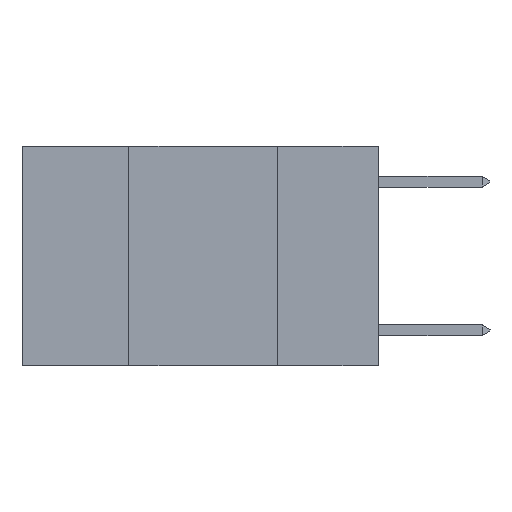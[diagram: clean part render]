
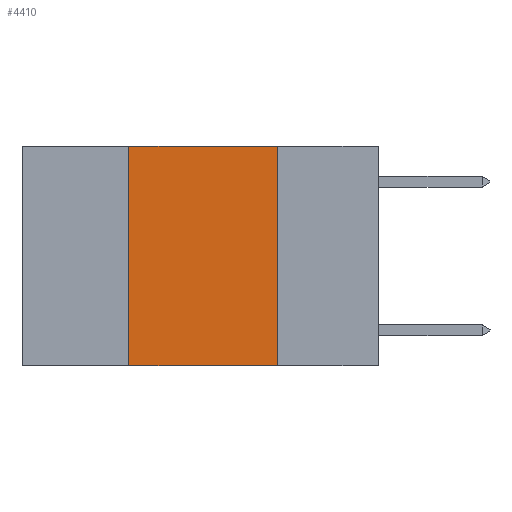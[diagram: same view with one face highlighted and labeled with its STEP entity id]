
A CAD part, left-side view. The second image highlights one B-rep face of the part: STEP entity #4410.
In plain terms, the highlighted planar face has unit normal (-1, 0, 0).
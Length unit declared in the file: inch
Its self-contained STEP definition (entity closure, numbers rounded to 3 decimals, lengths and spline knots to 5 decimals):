
#811 = VERTEX_POINT ( 'NONE', #2600 ) ;
#823 = DIRECTION ( 'NONE',  ( 0., 0., -1. ) ) ;
#842 = VECTOR ( 'NONE', #6022, 39.37008 ) ;
#880 = AXIS2_PLACEMENT_3D ( 'NONE', #5152, #6126, #823 ) ;
#996 = LINE ( 'NONE', #3697, #5371 ) ;
#1858 = VECTOR ( 'NONE', #10488, 39.37008 ) ;
#2410 = VECTOR ( 'NONE', #9389, 39.37008 ) ;
#2423 = VERTEX_POINT ( 'NONE', #10660 ) ;
#2434 = EDGE_CURVE ( 'NONE', #2423, #6472, #996, .T. ) ;
#2500 = EDGE_CURVE ( 'NONE', #811, #2423, #2654, .T. ) ;
#2600 = CARTESIAN_POINT ( 'NONE',  ( 0., 0.42, -0.37 ) ) ;
#2654 = LINE ( 'NONE', #4223, #2410 ) ;
#2968 = VERTEX_POINT ( 'NONE', #3787 ) ;
#3271 = EDGE_CURVE ( 'NONE', #811, #2968, #7727, .T. ) ;
#3697 = CARTESIAN_POINT ( 'NONE',  ( 0., 0.6, 0. ) ) ;
#3787 = CARTESIAN_POINT ( 'NONE',  ( 0., 0.17, -0.37 ) ) ;
#4223 = CARTESIAN_POINT ( 'NONE',  ( 0., 0.42, 0. ) ) ;
#4410 = ADVANCED_FACE ( 'NONE', ( #5024 ), #8493, .F. ) ;
#5024 = FACE_OUTER_BOUND ( 'NONE', #6814, .T. ) ;
#5152 = CARTESIAN_POINT ( 'NONE',  ( 0., 0.6, 0. ) ) ;
#5371 = VECTOR ( 'NONE', #9566, 39.37008 ) ;
#6022 = DIRECTION ( 'NONE',  ( 0., -1., 0. ) ) ;
#6126 = DIRECTION ( 'NONE',  ( 1., 0., 0. ) ) ;
#6472 = VERTEX_POINT ( 'NONE', #7845 ) ;
#6723 = EDGE_CURVE ( 'NONE', #6472, #2968, #10813, .T. ) ;
#6814 = EDGE_LOOP ( 'NONE', ( #9332, #8508, #8942, #9829 ) ) ;
#7570 = CARTESIAN_POINT ( 'NONE',  ( 0., 0.6, -0.37 ) ) ;
#7727 = LINE ( 'NONE', #7570, #842 ) ;
#7845 = CARTESIAN_POINT ( 'NONE',  ( 0., 0.17, 0. ) ) ;
#8493 = PLANE ( 'NONE',  #880 ) ;
#8508 = ORIENTED_EDGE ( 'NONE', *, *, #2434, .F. ) ;
#8942 = ORIENTED_EDGE ( 'NONE', *, *, #2500, .F. ) ;
#9332 = ORIENTED_EDGE ( 'NONE', *, *, #6723, .F. ) ;
#9389 = DIRECTION ( 'NONE',  ( 0., 0., 1. ) ) ;
#9566 = DIRECTION ( 'NONE',  ( 0., -1., 0. ) ) ;
#9713 = CARTESIAN_POINT ( 'NONE',  ( 0., 0.17, 0. ) ) ;
#9829 = ORIENTED_EDGE ( 'NONE', *, *, #3271, .T. ) ;
#10488 = DIRECTION ( 'NONE',  ( 0., 0., -1. ) ) ;
#10660 = CARTESIAN_POINT ( 'NONE',  ( 0., 0.42, 0. ) ) ;
#10813 = LINE ( 'NONE', #9713, #1858 ) ;
